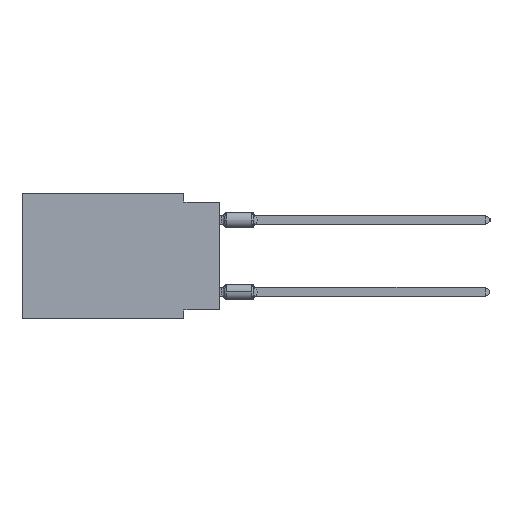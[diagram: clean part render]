
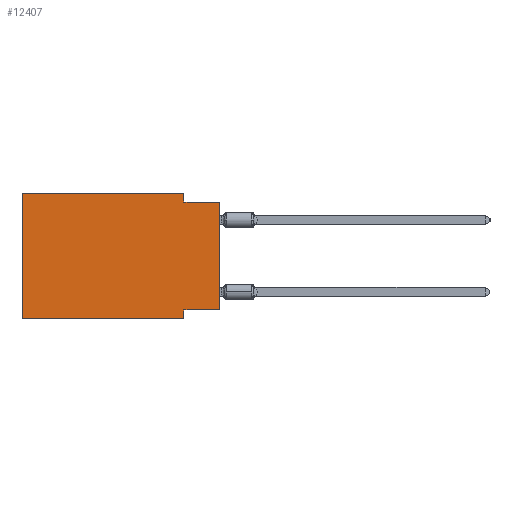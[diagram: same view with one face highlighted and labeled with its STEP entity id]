
A CAD part, left-side view. The second image highlights one B-rep face of the part: STEP entity #12407.
In plain terms, the highlighted planar face has unit normal (-1, 0, 0).
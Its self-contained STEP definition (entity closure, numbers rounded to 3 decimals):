
#421 = VECTOR ( 'NONE', #19149, 1000. ) ;
#1269 = VECTOR ( 'NONE', #29810, 1000. ) ;
#1669 = CARTESIAN_POINT ( 'NONE',  ( 0., 13.97, 0. ) ) ;
#2103 = DIRECTION ( 'NONE',  ( 0., -1., 0. ) ) ;
#2112 = VECTOR ( 'NONE', #34536, 1000. ) ;
#2145 = VERTEX_POINT ( 'NONE', #20949 ) ;
#2509 = DIRECTION ( 'NONE',  ( 0., -1., 0. ) ) ;
#3860 = CARTESIAN_POINT ( 'NONE',  ( 0., 2.54, 0. ) ) ;
#4067 = EDGE_CURVE ( 'NONE', #8753, #21306, #9600, .T. ) ;
#5869 = EDGE_CURVE ( 'NONE', #42136, #23738, #9144, .T. ) ;
#7224 = DIRECTION ( 'NONE',  ( 0., 1., 0. ) ) ;
#7642 = VECTOR ( 'NONE', #7224, 1000. ) ;
#8034 = CARTESIAN_POINT ( 'NONE',  ( 0., 2.54, -0.635 ) ) ;
#8068 = VECTOR ( 'NONE', #2509, 1000. ) ;
#8245 = AXIS2_PLACEMENT_3D ( 'NONE', #31497, #18274, #41028 ) ;
#8311 = PLANE ( 'NONE',  #8245 ) ;
#8526 = CARTESIAN_POINT ( 'NONE',  ( 0., 0., 0. ) ) ;
#8753 = VERTEX_POINT ( 'NONE', #3860 ) ;
#9144 = LINE ( 'NONE', #11752, #18409 ) ;
#9600 = LINE ( 'NONE', #39506, #421 ) ;
#11752 = CARTESIAN_POINT ( 'NONE',  ( 0., 13.97, 0. ) ) ;
#11880 = CARTESIAN_POINT ( 'NONE',  ( 0., 0., -8.255 ) ) ;
#12407 = ADVANCED_FACE ( 'NONE', ( #14806 ), #8311, .F. ) ;
#13227 = EDGE_CURVE ( 'NONE', #21306, #18036, #31808, .T. ) ;
#14496 = EDGE_CURVE ( 'NONE', #21826, #18036, #31085, .T. ) ;
#14806 = FACE_OUTER_BOUND ( 'NONE', #30119, .T. ) ;
#15822 = CARTESIAN_POINT ( 'NONE',  ( 0., 0., -0.635 ) ) ;
#16744 = VERTEX_POINT ( 'NONE', #19462 ) ;
#16788 = CARTESIAN_POINT ( 'NONE',  ( 0., 2.54, -8.89 ) ) ;
#18036 = VERTEX_POINT ( 'NONE', #15822 ) ;
#18274 = DIRECTION ( 'NONE',  ( 1., 0., 0. ) ) ;
#18409 = VECTOR ( 'NONE', #31687, 1000. ) ;
#19149 = DIRECTION ( 'NONE',  ( 0., 0., -1. ) ) ;
#19462 = CARTESIAN_POINT ( 'NONE',  ( 0., 2.54, -8.89 ) ) ;
#20050 = CARTESIAN_POINT ( 'NONE',  ( 0., 13.97, 0. ) ) ;
#20949 = CARTESIAN_POINT ( 'NONE',  ( 0., 2.54, -8.255 ) ) ;
#21306 = VERTEX_POINT ( 'NONE', #8034 ) ;
#21826 = VERTEX_POINT ( 'NONE', #11880 ) ;
#22276 = CARTESIAN_POINT ( 'NONE',  ( 0., 0., -0.635 ) ) ;
#22416 = VECTOR ( 'NONE', #27485, 1000. ) ;
#23689 = EDGE_CURVE ( 'NONE', #2145, #16744, #33046, .T. ) ;
#23738 = VERTEX_POINT ( 'NONE', #20050 ) ;
#27160 = LINE ( 'NONE', #36703, #7642 ) ;
#27314 = ORIENTED_EDGE ( 'NONE', *, *, #23689, .F. ) ;
#27485 = DIRECTION ( 'NONE',  ( 0., -1., 0. ) ) ;
#27582 = ORIENTED_EDGE ( 'NONE', *, *, #13227, .F. ) ;
#28397 = VECTOR ( 'NONE', #2103, 1000. ) ;
#28765 = CARTESIAN_POINT ( 'NONE',  ( 0., 13.97, -8.89 ) ) ;
#29770 = ORIENTED_EDGE ( 'NONE', *, *, #4067, .F. ) ;
#29810 = DIRECTION ( 'NONE',  ( 0., 0., -1. ) ) ;
#30119 = EDGE_LOOP ( 'NONE', ( #39744, #27582, #29770, #32859, #33482, #40577, #27314, #42649 ) ) ;
#31085 = LINE ( 'NONE', #8526, #2112 ) ;
#31497 = CARTESIAN_POINT ( 'NONE',  ( 0., 13.97, 0. ) ) ;
#31687 = DIRECTION ( 'NONE',  ( 0., 0., 1. ) ) ;
#31778 = EDGE_CURVE ( 'NONE', #23738, #8753, #34400, .T. ) ;
#31808 = LINE ( 'NONE', #22276, #28397 ) ;
#32859 = ORIENTED_EDGE ( 'NONE', *, *, #31778, .F. ) ;
#33046 = LINE ( 'NONE', #16788, #1269 ) ;
#33048 = CARTESIAN_POINT ( 'NONE',  ( 0., 13.97, -8.89 ) ) ;
#33482 = ORIENTED_EDGE ( 'NONE', *, *, #5869, .F. ) ;
#34400 = LINE ( 'NONE', #1669, #22416 ) ;
#34536 = DIRECTION ( 'NONE',  ( 0., 0., 1. ) ) ;
#35874 = EDGE_CURVE ( 'NONE', #42136, #16744, #42578, .T. ) ;
#36703 = CARTESIAN_POINT ( 'NONE',  ( 0., 0., -8.255 ) ) ;
#39506 = CARTESIAN_POINT ( 'NONE',  ( 0., 2.54, 0. ) ) ;
#39744 = ORIENTED_EDGE ( 'NONE', *, *, #14496, .T. ) ;
#40577 = ORIENTED_EDGE ( 'NONE', *, *, #35874, .T. ) ;
#41028 = DIRECTION ( 'NONE',  ( 0., 0., -1. ) ) ;
#42136 = VERTEX_POINT ( 'NONE', #28765 ) ;
#42578 = LINE ( 'NONE', #33048, #8068 ) ;
#42633 = EDGE_CURVE ( 'NONE', #21826, #2145, #27160, .T. ) ;
#42649 = ORIENTED_EDGE ( 'NONE', *, *, #42633, .F. ) ;
